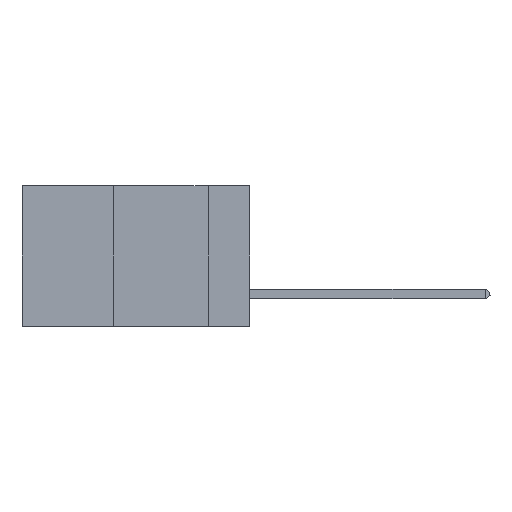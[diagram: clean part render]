
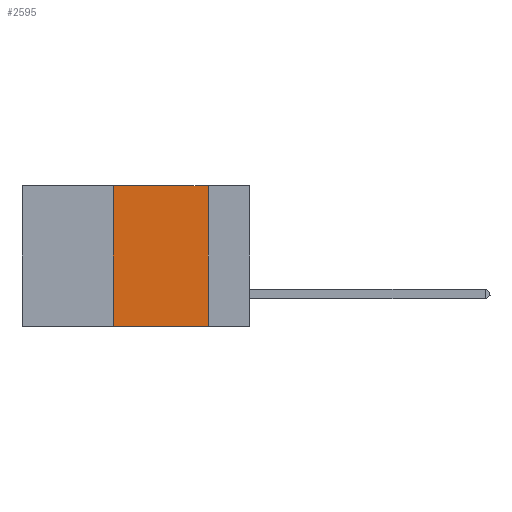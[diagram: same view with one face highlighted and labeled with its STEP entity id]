
A CAD part, left-side view. The second image highlights one B-rep face of the part: STEP entity #2595.
In plain terms, the highlighted planar face has unit normal (-1, 0, 0).
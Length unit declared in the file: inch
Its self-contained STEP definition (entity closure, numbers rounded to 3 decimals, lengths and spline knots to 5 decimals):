
#557 = VECTOR ( 'NONE', #18766, 39.37008 ) ;
#1046 = EDGE_CURVE ( 'NONE', #38755, #39899, #41680, .T. ) ;
#2595 = ADVANCED_FACE ( 'NONE', ( #28280 ), #31906, .F. ) ;
#2999 = ORIENTED_EDGE ( 'NONE', *, *, #17357, .F. ) ;
#3935 = EDGE_CURVE ( 'NONE', #34610, #39899, #37308, .T. ) ;
#4440 = VERTEX_POINT ( 'NONE', #31548 ) ;
#5046 = CARTESIAN_POINT ( 'NONE',  ( 0., 0.11, -0.37 ) ) ;
#6640 = CARTESIAN_POINT ( 'NONE',  ( 0., 0.11, 0. ) ) ;
#8133 = VECTOR ( 'NONE', #24800, 39.37008 ) ;
#8774 = CARTESIAN_POINT ( 'NONE',  ( 0., 0.6, -0.37 ) ) ;
#8864 = ORIENTED_EDGE ( 'NONE', *, *, #1046, .F. ) ;
#12089 = VECTOR ( 'NONE', #41860, 39.37008 ) ;
#12258 = CARTESIAN_POINT ( 'NONE',  ( 0., 0.6, 0. ) ) ;
#15577 = LINE ( 'NONE', #12258, #25795 ) ;
#16485 = CARTESIAN_POINT ( 'NONE',  ( 0., 0.6, 0. ) ) ;
#17357 = EDGE_CURVE ( 'NONE', #4440, #38755, #15577, .T. ) ;
#17921 = CARTESIAN_POINT ( 'NONE',  ( 0., 0.36, 0. ) ) ;
#18625 = CARTESIAN_POINT ( 'NONE',  ( 0., 0.36, -0.37 ) ) ;
#18766 = DIRECTION ( 'NONE',  ( 0., -1., 0. ) ) ;
#19459 = EDGE_LOOP ( 'NONE', ( #8864, #2999, #27129, #20874 ) ) ;
#20874 = ORIENTED_EDGE ( 'NONE', *, *, #3935, .T. ) ;
#22586 = EDGE_CURVE ( 'NONE', #34610, #4440, #34172, .T. ) ;
#24800 = DIRECTION ( 'NONE',  ( 0., 0., 1. ) ) ;
#25130 = CARTESIAN_POINT ( 'NONE',  ( 0., 0.11, 0. ) ) ;
#25795 = VECTOR ( 'NONE', #41930, 39.37008 ) ;
#27129 = ORIENTED_EDGE ( 'NONE', *, *, #22586, .F. ) ;
#28280 = FACE_OUTER_BOUND ( 'NONE', #19459, .T. ) ;
#31000 = DIRECTION ( 'NONE',  ( 1., 0., 0. ) ) ;
#31548 = CARTESIAN_POINT ( 'NONE',  ( 0., 0.36, 0. ) ) ;
#31906 = PLANE ( 'NONE',  #37741 ) ;
#34172 = LINE ( 'NONE', #17921, #8133 ) ;
#34610 = VERTEX_POINT ( 'NONE', #18625 ) ;
#37308 = LINE ( 'NONE', #8774, #557 ) ;
#37741 = AXIS2_PLACEMENT_3D ( 'NONE', #16485, #31000, #39680 ) ;
#38755 = VERTEX_POINT ( 'NONE', #25130 ) ;
#39680 = DIRECTION ( 'NONE',  ( 0., 0., -1. ) ) ;
#39899 = VERTEX_POINT ( 'NONE', #5046 ) ;
#41680 = LINE ( 'NONE', #6640, #12089 ) ;
#41860 = DIRECTION ( 'NONE',  ( 0., 0., -1. ) ) ;
#41930 = DIRECTION ( 'NONE',  ( 0., -1., 0. ) ) ;
